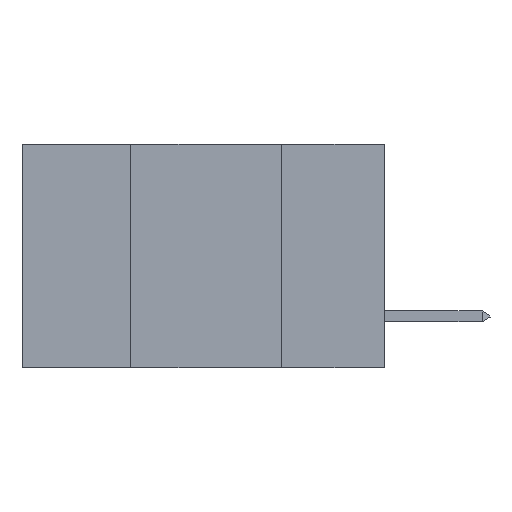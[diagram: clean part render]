
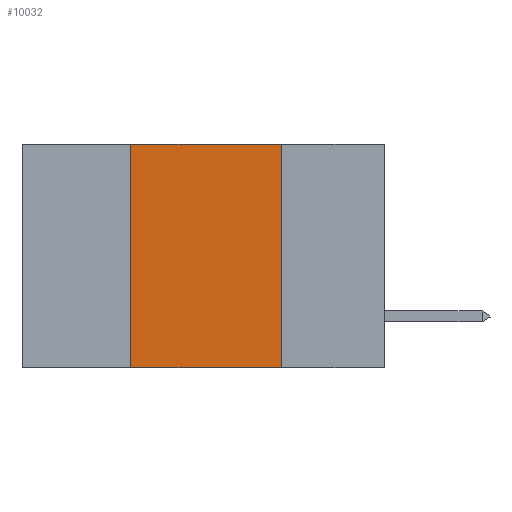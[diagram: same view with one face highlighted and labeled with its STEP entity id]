
A CAD part, left-side view. The second image highlights one B-rep face of the part: STEP entity #10032.
In plain terms, the highlighted planar face has unit normal (-1, 0, 0).
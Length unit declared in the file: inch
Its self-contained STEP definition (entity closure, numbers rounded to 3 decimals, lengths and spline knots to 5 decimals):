
#2475 = EDGE_CURVE ( 'NONE', #12080, #18602, #45605, .T. ) ;
#3418 = CARTESIAN_POINT ( 'NONE',  ( 0., 0.42, -0.37 ) ) ;
#6560 = DIRECTION ( 'NONE',  ( 0., 0., -1. ) ) ;
#8041 = CARTESIAN_POINT ( 'NONE',  ( 0., 0.6, 0. ) ) ;
#8693 = ORIENTED_EDGE ( 'NONE', *, *, #25988, .F. ) ;
#8836 = DIRECTION ( 'NONE',  ( 1., 0., 0. ) ) ;
#9580 = AXIS2_PLACEMENT_3D ( 'NONE', #8041, #8836, #37853 ) ;
#9612 = CARTESIAN_POINT ( 'NONE',  ( 0., 0.6, 0. ) ) ;
#10032 = ADVANCED_FACE ( 'NONE', ( #41559 ), #44962, .F. ) ;
#10048 = LINE ( 'NONE', #9612, #27337 ) ;
#10093 = CARTESIAN_POINT ( 'NONE',  ( 0., 0.17, 0. ) ) ;
#12080 = VERTEX_POINT ( 'NONE', #3418 ) ;
#14609 = VERTEX_POINT ( 'NONE', #26444 ) ;
#14992 = CARTESIAN_POINT ( 'NONE',  ( 0., 0.17, -0.37 ) ) ;
#15993 = ORIENTED_EDGE ( 'NONE', *, *, #2475, .F. ) ;
#16571 = ORIENTED_EDGE ( 'NONE', *, *, #45608, .F. ) ;
#18602 = VERTEX_POINT ( 'NONE', #42552 ) ;
#23602 = ORIENTED_EDGE ( 'NONE', *, *, #41642, .T. ) ;
#24096 = DIRECTION ( 'NONE',  ( 0., -1., 0. ) ) ;
#25347 = LINE ( 'NONE', #46181, #47397 ) ;
#25988 = EDGE_CURVE ( 'NONE', #18602, #14609, #10048, .T. ) ;
#26444 = CARTESIAN_POINT ( 'NONE',  ( 0., 0.17, 0. ) ) ;
#27337 = VECTOR ( 'NONE', #24096, 39.37008 ) ;
#29296 = EDGE_LOOP ( 'NONE', ( #16571, #8693, #15993, #23602 ) ) ;
#30804 = LINE ( 'NONE', #10093, #33732 ) ;
#33462 = CARTESIAN_POINT ( 'NONE',  ( 0., 0.42, 0. ) ) ;
#33732 = VECTOR ( 'NONE', #6560, 39.37008 ) ;
#36674 = DIRECTION ( 'NONE',  ( 0., -1., 0. ) ) ;
#37853 = DIRECTION ( 'NONE',  ( 0., 0., -1. ) ) ;
#40951 = DIRECTION ( 'NONE',  ( 0., 0., 1. ) ) ;
#41559 = FACE_OUTER_BOUND ( 'NONE', #29296, .T. ) ;
#41642 = EDGE_CURVE ( 'NONE', #12080, #45776, #25347, .T. ) ;
#42552 = CARTESIAN_POINT ( 'NONE',  ( 0., 0.42, 0. ) ) ;
#44962 = PLANE ( 'NONE',  #9580 ) ;
#45605 = LINE ( 'NONE', #33462, #47394 ) ;
#45608 = EDGE_CURVE ( 'NONE', #14609, #45776, #30804, .T. ) ;
#45776 = VERTEX_POINT ( 'NONE', #14992 ) ;
#46181 = CARTESIAN_POINT ( 'NONE',  ( 0., 0.6, -0.37 ) ) ;
#47394 = VECTOR ( 'NONE', #40951, 39.37008 ) ;
#47397 = VECTOR ( 'NONE', #36674, 39.37008 ) ;
